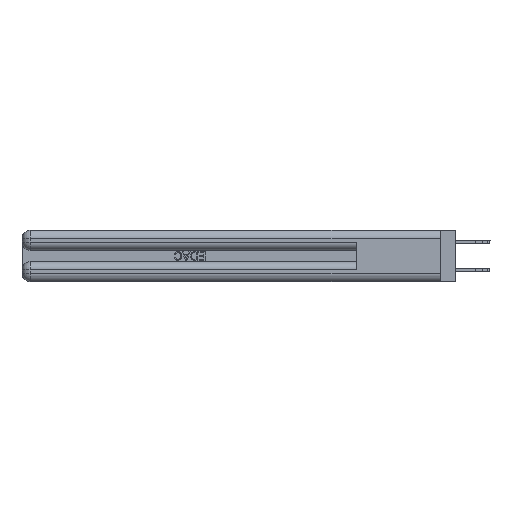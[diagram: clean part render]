
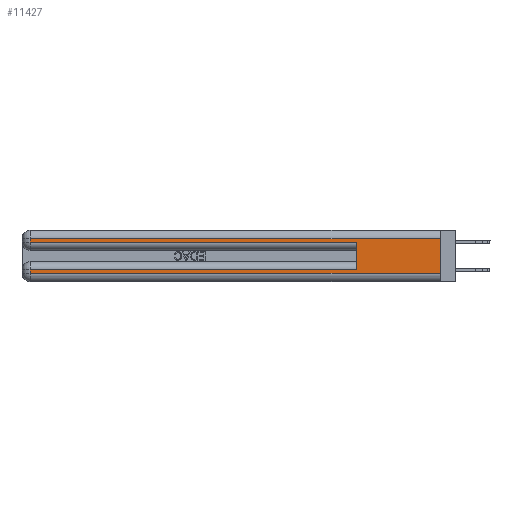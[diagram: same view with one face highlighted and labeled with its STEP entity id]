
A CAD part, left-side view. The second image highlights one B-rep face of the part: STEP entity #11427.
In plain terms, the highlighted planar face has unit normal (-1, 0, 0).
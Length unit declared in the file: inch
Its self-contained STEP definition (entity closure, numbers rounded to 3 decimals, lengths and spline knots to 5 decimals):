
#78 = ORIENTED_EDGE ( 'NONE', *, *, #3735, .T. ) ;
#3735 = EDGE_CURVE ( 'NONE', #25261, #20488, #34317, .T. ) ;
#3829 = DIRECTION ( 'NONE',  ( 0., 1., 0. ) ) ;
#5452 = CARTESIAN_POINT ( 'NONE',  ( 0., 2.94, 0.37 ) ) ;
#5610 = VECTOR ( 'NONE', #36527, 39.37008 ) ;
#6043 = LINE ( 'NONE', #13576, #29974 ) ;
#6612 = VECTOR ( 'NONE', #11324, 39.37008 ) ;
#8804 = FACE_OUTER_BOUND ( 'NONE', #29399, .T. ) ;
#10159 = DIRECTION ( 'NONE',  ( 0., 0., -1. ) ) ;
#10193 = VECTOR ( 'NONE', #3829, 39.37008 ) ;
#11324 = DIRECTION ( 'NONE',  ( 0., 0., -1. ) ) ;
#11427 = ADVANCED_FACE ( 'NONE', ( #8804 ), #25371, .F. ) ;
#11687 = EDGE_CURVE ( 'NONE', #27382, #35078, #26108, .T. ) ;
#12879 = VECTOR ( 'NONE', #17738, 39.37008 ) ;
#13085 = ORIENTED_EDGE ( 'NONE', *, *, #15896, .T. ) ;
#13179 = VERTEX_POINT ( 'NONE', #30884 ) ;
#13244 = VECTOR ( 'NONE', #37993, 39.37008 ) ;
#13576 = CARTESIAN_POINT ( 'NONE',  ( 0., 0., 0.31 ) ) ;
#13584 = CARTESIAN_POINT ( 'NONE',  ( 0., 0., 0.37 ) ) ;
#14874 = ORIENTED_EDGE ( 'NONE', *, *, #21743, .T. ) ;
#14961 = CARTESIAN_POINT ( 'NONE',  ( 0., 0., 0.31 ) ) ;
#15550 = EDGE_CURVE ( 'NONE', #20488, #26605, #29477, .T. ) ;
#15896 = EDGE_CURVE ( 'NONE', #32299, #13179, #35597, .T. ) ;
#16851 = CARTESIAN_POINT ( 'NONE',  ( 0., 2.94, 0.31 ) ) ;
#17137 = ORIENTED_EDGE ( 'NONE', *, *, #15550, .T. ) ;
#17544 = CARTESIAN_POINT ( 'NONE',  ( 0., 0.6, 0.085 ) ) ;
#17738 = DIRECTION ( 'NONE',  ( 0., 0., 1. ) ) ;
#18001 = ORIENTED_EDGE ( 'NONE', *, *, #11687, .F. ) ;
#18578 = CARTESIAN_POINT ( 'NONE',  ( 0., 0., 0.06 ) ) ;
#19091 = ORIENTED_EDGE ( 'NONE', *, *, #24073, .F. ) ;
#19207 = DIRECTION ( 'NONE',  ( 1., 0., 0. ) ) ;
#19900 = LINE ( 'NONE', #23918, #12879 ) ;
#20100 = DIRECTION ( 'NONE',  ( 0., 1., 0. ) ) ;
#20488 = VERTEX_POINT ( 'NONE', #30467 ) ;
#21620 = EDGE_CURVE ( 'NONE', #33443, #35078, #21990, .T. ) ;
#21743 = EDGE_CURVE ( 'NONE', #27382, #25261, #6043, .T. ) ;
#21990 = LINE ( 'NONE', #30837, #5610 ) ;
#22115 = DIRECTION ( 'NONE',  ( 0., -1., 0. ) ) ;
#23918 = CARTESIAN_POINT ( 'NONE',  ( 0., 0.6, 0.145 ) ) ;
#24073 = EDGE_CURVE ( 'NONE', #32299, #26605, #19900, .T. ) ;
#24320 = CARTESIAN_POINT ( 'NONE',  ( 0., 0., 0.085 ) ) ;
#24993 = LINE ( 'NONE', #5452, #13244 ) ;
#25261 = VERTEX_POINT ( 'NONE', #16851 ) ;
#25371 = PLANE ( 'NONE',  #36475 ) ;
#25803 = CARTESIAN_POINT ( 'NONE',  ( 0., 0.6, 0.285 ) ) ;
#26108 = LINE ( 'NONE', #13584, #27976 ) ;
#26605 = VERTEX_POINT ( 'NONE', #25803 ) ;
#27382 = VERTEX_POINT ( 'NONE', #14961 ) ;
#27971 = ORIENTED_EDGE ( 'NONE', *, *, #21620, .T. ) ;
#27976 = VECTOR ( 'NONE', #32445, 39.37008 ) ;
#28259 = CARTESIAN_POINT ( 'NONE',  ( 0., 0., 0.285 ) ) ;
#29399 = EDGE_LOOP ( 'NONE', ( #18001, #14874, #78, #17137, #19091, #13085, #34299, #27971 ) ) ;
#29477 = LINE ( 'NONE', #28259, #29962 ) ;
#29962 = VECTOR ( 'NONE', #22115, 39.37008 ) ;
#29974 = VECTOR ( 'NONE', #20100, 39.37008 ) ;
#30467 = CARTESIAN_POINT ( 'NONE',  ( 0., 2.94, 0.285 ) ) ;
#30811 = EDGE_CURVE ( 'NONE', #13179, #33443, #24993, .T. ) ;
#30837 = CARTESIAN_POINT ( 'NONE',  ( 0., 0., 0.06 ) ) ;
#30884 = CARTESIAN_POINT ( 'NONE',  ( 0., 2.94, 0.085 ) ) ;
#32299 = VERTEX_POINT ( 'NONE', #17544 ) ;
#32445 = DIRECTION ( 'NONE',  ( 0., 0., -1. ) ) ;
#33443 = VERTEX_POINT ( 'NONE', #38435 ) ;
#34299 = ORIENTED_EDGE ( 'NONE', *, *, #30811, .T. ) ;
#34317 = LINE ( 'NONE', #35211, #6612 ) ;
#35078 = VERTEX_POINT ( 'NONE', #18578 ) ;
#35211 = CARTESIAN_POINT ( 'NONE',  ( 0., 2.94, 0.37 ) ) ;
#35597 = LINE ( 'NONE', #24320, #10193 ) ;
#36475 = AXIS2_PLACEMENT_3D ( 'NONE', #37344, #19207, #10159 ) ;
#36527 = DIRECTION ( 'NONE',  ( 0., -1., 0. ) ) ;
#37344 = CARTESIAN_POINT ( 'NONE',  ( 0., 0., 0.37 ) ) ;
#37993 = DIRECTION ( 'NONE',  ( 0., 0., -1. ) ) ;
#38435 = CARTESIAN_POINT ( 'NONE',  ( 0., 2.94, 0.06 ) ) ;
